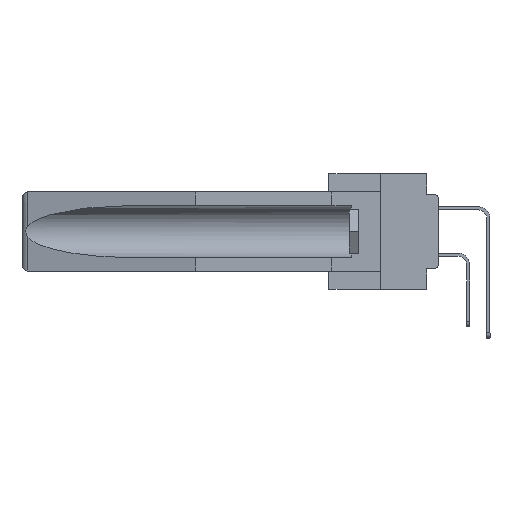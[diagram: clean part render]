
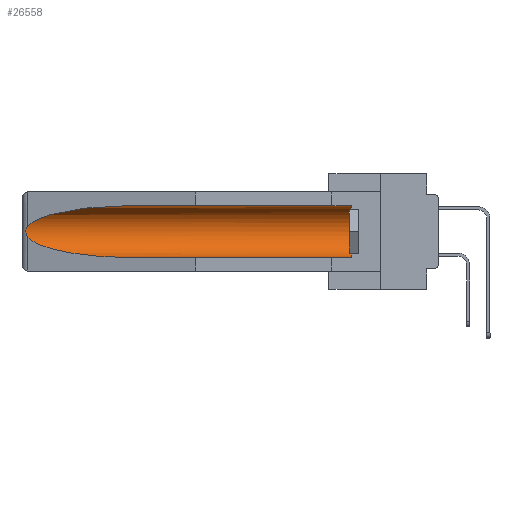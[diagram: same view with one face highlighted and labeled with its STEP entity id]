
A CAD part, left-side view. The second image highlights one B-rep face of the part: STEP entity #26558.
In plain terms, the highlighted cylindrical face has radius 2.857 mm (diameter 5.715 mm), a partial arc.
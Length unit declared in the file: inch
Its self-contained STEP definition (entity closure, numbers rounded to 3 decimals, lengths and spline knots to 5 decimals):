
#132 = CYLINDRICAL_SURFACE ( 'NONE', #16858, 0.1125 ) ;
#293 = CARTESIAN_POINT ( 'NONE',  ( 0.2673, 1.5327, -0.16383 ) ) ;
#470 = CARTESIAN_POINT ( 'NONE',  ( 0.2675, 1.53308, -0.17534 ) ) ;
#1882 = LINE ( 'NONE', #2239, #18505 ) ;
#1894 = ORIENTED_EDGE ( 'NONE', *, *, #21688, .T. ) ;
#2061 = DIRECTION ( 'NONE',  ( 0., 1., 0. ) ) ;
#2239 = CARTESIAN_POINT ( 'NONE',  ( 0.155, -0.30754, -0.059 ) ) ;
#2338 = CARTESIAN_POINT ( 'NONE',  ( 0.155, 1.07973, -0.284 ) ) ;
#2375 = CARTESIAN_POINT ( 'NONE',  ( 0.26537, 1.52718, -0.14972 ) ) ;
#3343 = CARTESIAN_POINT ( 'NONE',  ( 0.21114, 1.30732, -0.284 ) ) ;
#3356 = CARTESIAN_POINT ( 'NONE',  ( 0.26537, 1.52718, -0.14972 ) ) ;
#5288 = CARTESIAN_POINT ( 'NONE',  ( 0.155, 0.126, -0.1715 ) ) ;
#5573 = DIRECTION ( 'NONE',  ( 0., 0., 1. ) ) ;
#5731 = CARTESIAN_POINT ( 'NONE',  ( 0.26597, 1.52961, -0.15275 ) ) ;
#6292 = CARTESIAN_POINT ( 'NONE',  ( 0.155, -0.30754, -0.1715 ) ) ;
#8445 = CARTESIAN_POINT ( 'NONE',  ( 0.25451, 1.48313, -0.09465 ) ) ;
#10077 = VECTOR ( 'NONE', #19787, 39.37008 ) ;
#10092 = CARTESIAN_POINT ( 'NONE',  ( 0.155, 1.07973, -0.059 ) ) ;
#11172 = CARTESIAN_POINT ( 'NONE',  ( 0.26537, 1.52718, -0.19328 ) ) ;
#11369 = CARTESIAN_POINT ( 'NONE',  ( 0.2675, 1.53308, -0.16763 ) ) ;
#11521 = CARTESIAN_POINT ( 'NONE',  ( 0.21114, 1.30732, -0.059 ) ) ;
#12004 = EDGE_CURVE ( 'NONE', #26958, #17653, #28222, .T. ) ;
#12241 =( BOUNDED_CURVE ( )  B_SPLINE_CURVE ( 3, ( #30648, #11521, #8445, #27367 ),
 .UNSPECIFIED., .F., .F. ) 
 B_SPLINE_CURVE_WITH_KNOTS ( ( 4, 4 ),
 ( 4.71239, 6.08839 ),
 .UNSPECIFIED. ) 
 CURVE ( )  GEOMETRIC_REPRESENTATION_ITEM ( )  RATIONAL_B_SPLINE_CURVE ( ( 1., 0.848, 0.848, 1. ) ) 
 REPRESENTATION_ITEM ( '' )  );
#12529 = AXIS2_PLACEMENT_3D ( 'NONE', #5288, #16046, #24596 ) ;
#14467 = CARTESIAN_POINT ( 'NONE',  ( 0.26537, 1.52718, -0.19328 ) ) ;
#14853 = EDGE_CURVE ( 'NONE', #30176, #18370, #12241, .T. ) ;
#15021 = CARTESIAN_POINT ( 'NONE',  ( 0.155, 0.126, -0.059 ) ) ;
#15803 = CARTESIAN_POINT ( 'NONE',  ( 0.26537, 1.52718, -0.19328 ) ) ;
#16046 = DIRECTION ( 'NONE',  ( 0., -1., 0. ) ) ;
#16858 = AXIS2_PLACEMENT_3D ( 'NONE', #6292, #28496, #5573 ) ;
#17215 = CARTESIAN_POINT ( 'NONE',  ( 0.26655, 1.53094, -0.18657 ) ) ;
#17242 = CARTESIAN_POINT ( 'NONE',  ( 0.155, -0.30754, -0.284 ) ) ;
#17416 = FACE_OUTER_BOUND ( 'NONE', #28571, .T. ) ;
#17619 = EDGE_CURVE ( 'NONE', #18370, #33720, #26457, .T. ) ;
#17653 = VERTEX_POINT ( 'NONE', #15021 ) ;
#18370 = VERTEX_POINT ( 'NONE', #2375 ) ;
#18505 = VECTOR ( 'NONE', #2061, 39.37008 ) ;
#19486 =( BOUNDED_CURVE ( )  B_SPLINE_CURVE ( 3, ( #11172, #22312, #3343, #33377 ),
 .UNSPECIFIED., .F., .F. ) 
 B_SPLINE_CURVE_WITH_KNOTS ( ( 4, 4 ),
 ( 0.1948, 1.5708 ),
 .UNSPECIFIED. ) 
 CURVE ( )  GEOMETRIC_REPRESENTATION_ITEM ( )  RATIONAL_B_SPLINE_CURVE ( ( 1., 0.848, 0.848, 1. ) ) 
 REPRESENTATION_ITEM ( '' )  );
#19787 = DIRECTION ( 'NONE',  ( 0., 1., 0. ) ) ;
#19978 = VERTEX_POINT ( 'NONE', #2338 ) ;
#21290 = ORIENTED_EDGE ( 'NONE', *, *, #29970, .F. ) ;
#21688 = EDGE_CURVE ( 'NONE', #33720, #19978, #19486, .T. ) ;
#22312 = CARTESIAN_POINT ( 'NONE',  ( 0.25451, 1.48313, -0.24835 ) ) ;
#22507 = CARTESIAN_POINT ( 'NONE',  ( 0.2673, 1.53269, -0.17917 ) ) ;
#22784 = ORIENTED_EDGE ( 'NONE', *, *, #23265, .T. ) ;
#23265 = EDGE_CURVE ( 'NONE', #17653, #30176, #1882, .T. ) ;
#24596 = DIRECTION ( 'NONE',  ( 0., 0., 1. ) ) ;
#25236 = LINE ( 'NONE', #17242, #10077 ) ;
#25501 = CARTESIAN_POINT ( 'NONE',  ( 0.155, 0.126, -0.284 ) ) ;
#25655 = ORIENTED_EDGE ( 'NONE', *, *, #17619, .T. ) ;
#26457 = B_SPLINE_CURVE_WITH_KNOTS ( 'NONE', 3,
 ( #3356, #5731, #31029, #293, #11369, #470, #22507, #17215, #28292, #14467 ),
 .UNSPECIFIED., .F., .F.,
 ( 4, 2, 2, 2, 4 ),
 ( 0., 0.00029, 0.00058, 0.00087, 0.00117 ),
 .UNSPECIFIED. ) ;
#26558 = ADVANCED_FACE ( 'NONE', ( #17416 ), #132, .F. ) ;
#26958 = VERTEX_POINT ( 'NONE', #25501 ) ;
#27367 = CARTESIAN_POINT ( 'NONE',  ( 0.26537, 1.52718, -0.14972 ) ) ;
#28222 = CIRCLE ( 'NONE', #12529, 0.1125 ) ;
#28292 = CARTESIAN_POINT ( 'NONE',  ( 0.26597, 1.5296, -0.19026 ) ) ;
#28418 = ORIENTED_EDGE ( 'NONE', *, *, #12004, .T. ) ;
#28496 = DIRECTION ( 'NONE',  ( 0., 1., 0. ) ) ;
#28511 = ORIENTED_EDGE ( 'NONE', *, *, #14853, .T. ) ;
#28571 = EDGE_LOOP ( 'NONE', ( #28511, #25655, #1894, #21290, #28418, #22784 ) ) ;
#29970 = EDGE_CURVE ( 'NONE', #26958, #19978, #25236, .T. ) ;
#30176 = VERTEX_POINT ( 'NONE', #10092 ) ;
#30648 = CARTESIAN_POINT ( 'NONE',  ( 0.155, 1.07973, -0.059 ) ) ;
#31029 = CARTESIAN_POINT ( 'NONE',  ( 0.26654, 1.53092, -0.15636 ) ) ;
#33377 = CARTESIAN_POINT ( 'NONE',  ( 0.155, 1.07973, -0.284 ) ) ;
#33720 = VERTEX_POINT ( 'NONE', #15803 ) ;
